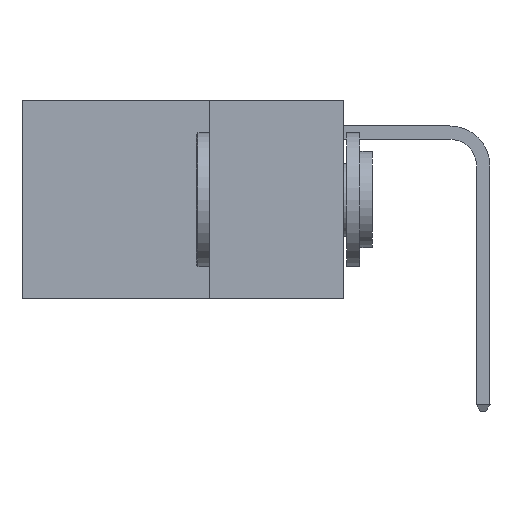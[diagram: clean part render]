
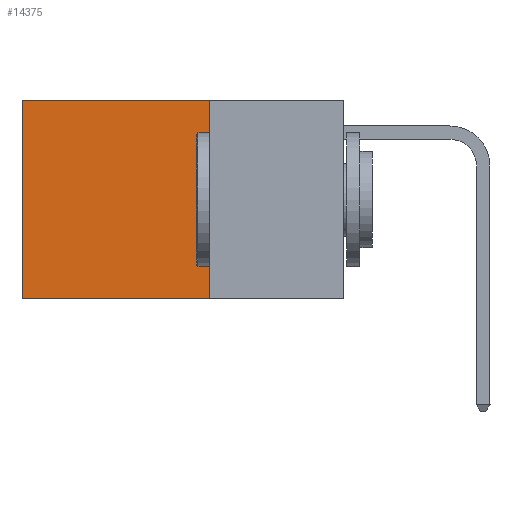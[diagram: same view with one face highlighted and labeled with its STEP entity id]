
A CAD part, left-side view. The second image highlights one B-rep face of the part: STEP entity #14375.
In plain terms, the highlighted planar face has unit normal (-1, 0, 0).
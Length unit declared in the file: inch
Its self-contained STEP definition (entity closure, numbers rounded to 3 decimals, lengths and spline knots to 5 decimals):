
#1039 = ORIENTED_EDGE ( 'NONE', *, *, #3013, .T. ) ;
#1236 = VERTEX_POINT ( 'NONE', #10135 ) ;
#1671 = CARTESIAN_POINT ( 'NONE',  ( 0.2625, 0.25, 0. ) ) ;
#3013 = EDGE_CURVE ( 'NONE', #10024, #12704, #22230, .T. ) ;
#3135 = ORIENTED_EDGE ( 'NONE', *, *, #10019, .F. ) ;
#5047 = CARTESIAN_POINT ( 'NONE',  ( 0.2625, 0.25, 0. ) ) ;
#5559 = ORIENTED_EDGE ( 'NONE', *, *, #12300, .T. ) ;
#6694 = FACE_OUTER_BOUND ( 'NONE', #23119, .T. ) ;
#7436 = CARTESIAN_POINT ( 'NONE',  ( 0.2625, 0.25, -0.37 ) ) ;
#7817 = PLANE ( 'NONE',  #12827 ) ;
#8100 = VECTOR ( 'NONE', #14328, 39.37008 ) ;
#8557 = EDGE_CURVE ( 'NONE', #17105, #1236, #10643, .T. ) ;
#8713 = LINE ( 'NONE', #12308, #8100 ) ;
#10019 = EDGE_CURVE ( 'NONE', #1236, #12704, #16837, .T. ) ;
#10024 = VERTEX_POINT ( 'NONE', #25351 ) ;
#10135 = CARTESIAN_POINT ( 'NONE',  ( 0.2625, 0.25, -0.37 ) ) ;
#10643 = LINE ( 'NONE', #1671, #25833 ) ;
#11476 = VECTOR ( 'NONE', #19413, 39.37008 ) ;
#11583 = CARTESIAN_POINT ( 'NONE',  ( 0.2625, 0.6, -0.37 ) ) ;
#11845 = DIRECTION ( 'NONE',  ( 0., 0., -1. ) ) ;
#12300 = EDGE_CURVE ( 'NONE', #17105, #10024, #8713, .T. ) ;
#12308 = CARTESIAN_POINT ( 'NONE',  ( 0.2625, 0.25, 0. ) ) ;
#12704 = VERTEX_POINT ( 'NONE', #11583 ) ;
#12827 = AXIS2_PLACEMENT_3D ( 'NONE', #21813, #23773, #11845 ) ;
#14328 = DIRECTION ( 'NONE',  ( 0., 1., 0. ) ) ;
#14375 = ADVANCED_FACE ( 'NONE', ( #6694 ), #7817, .F. ) ;
#15893 = ORIENTED_EDGE ( 'NONE', *, *, #8557, .F. ) ;
#16837 = LINE ( 'NONE', #7436, #11476 ) ;
#16930 = VECTOR ( 'NONE', #24543, 39.37008 ) ;
#17105 = VERTEX_POINT ( 'NONE', #5047 ) ;
#17690 = DIRECTION ( 'NONE',  ( 0., 0., -1. ) ) ;
#19413 = DIRECTION ( 'NONE',  ( 0., 1., 0. ) ) ;
#20547 = CARTESIAN_POINT ( 'NONE',  ( 0.2625, 0.6, 0. ) ) ;
#21813 = CARTESIAN_POINT ( 'NONE',  ( 0.2625, 0.25, 0. ) ) ;
#22230 = LINE ( 'NONE', #20547, #16930 ) ;
#23119 = EDGE_LOOP ( 'NONE', ( #1039, #3135, #15893, #5559 ) ) ;
#23773 = DIRECTION ( 'NONE',  ( 1., 0., 0. ) ) ;
#24543 = DIRECTION ( 'NONE',  ( 0., 0., -1. ) ) ;
#25351 = CARTESIAN_POINT ( 'NONE',  ( 0.2625, 0.6, 0. ) ) ;
#25833 = VECTOR ( 'NONE', #17690, 39.37008 ) ;
